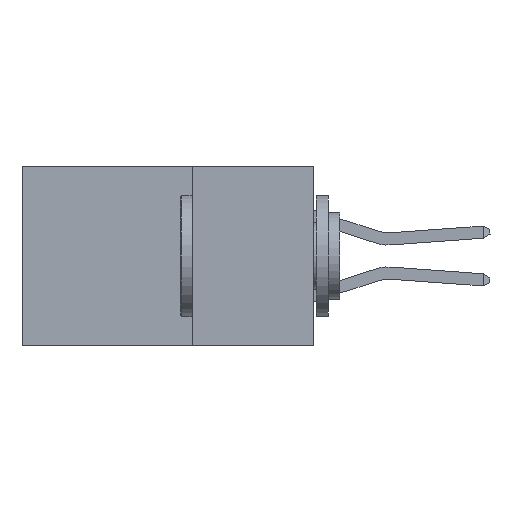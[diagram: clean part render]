
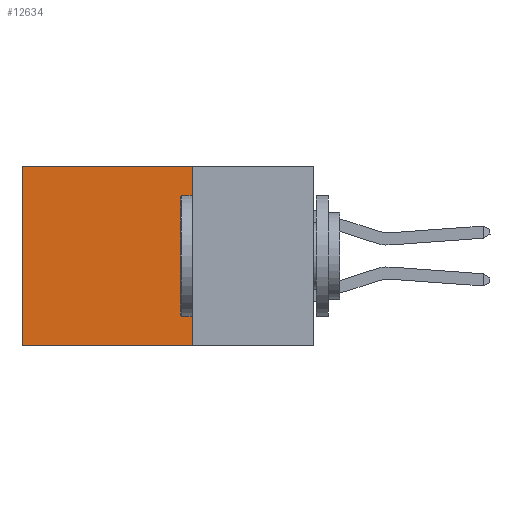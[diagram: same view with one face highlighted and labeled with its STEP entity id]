
A CAD part, left-side view. The second image highlights one B-rep face of the part: STEP entity #12634.
In plain terms, the highlighted planar face has unit normal (-1, 0, 0).
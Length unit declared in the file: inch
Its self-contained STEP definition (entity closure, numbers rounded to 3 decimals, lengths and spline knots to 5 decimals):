
#75 = DIRECTION ( 'NONE',  ( 0., 0., -1. ) ) ;
#630 = LINE ( 'NONE', #6288, #9012 ) ;
#951 = VECTOR ( 'NONE', #9640, 39.37008 ) ;
#1328 = EDGE_CURVE ( 'NONE', #14599, #2252, #17399, .T. ) ;
#1949 = LINE ( 'NONE', #2271, #10211 ) ;
#1964 = FACE_OUTER_BOUND ( 'NONE', #18501, .T. ) ;
#2252 = VERTEX_POINT ( 'NONE', #11704 ) ;
#2271 = CARTESIAN_POINT ( 'NONE',  ( 0.2875, 0.25, -0.37 ) ) ;
#3451 = PLANE ( 'NONE',  #10579 ) ;
#4205 = EDGE_CURVE ( 'NONE', #14599, #5787, #630, .T. ) ;
#4872 = VERTEX_POINT ( 'NONE', #7688 ) ;
#5141 = DIRECTION ( 'NONE',  ( 1., 0., 0. ) ) ;
#5209 = CARTESIAN_POINT ( 'NONE',  ( 0.2875, 0.25, 0. ) ) ;
#5787 = VERTEX_POINT ( 'NONE', #16087 ) ;
#6288 = CARTESIAN_POINT ( 'NONE',  ( 0.2875, 0.25, 0. ) ) ;
#6565 = DIRECTION ( 'NONE',  ( 0., 1., 0. ) ) ;
#7688 = CARTESIAN_POINT ( 'NONE',  ( 0.2875, 0.6, -0.37 ) ) ;
#8024 = CARTESIAN_POINT ( 'NONE',  ( 0.2875, 0.6, 0. ) ) ;
#9012 = VECTOR ( 'NONE', #6565, 39.37008 ) ;
#9640 = DIRECTION ( 'NONE',  ( 0., 0., -1. ) ) ;
#9945 = ORIENTED_EDGE ( 'NONE', *, *, #9954, .T. ) ;
#9954 = EDGE_CURVE ( 'NONE', #5787, #4872, #13933, .T. ) ;
#9970 = CARTESIAN_POINT ( 'NONE',  ( 0.2875, 0.25, 0. ) ) ;
#10211 = VECTOR ( 'NONE', #15088, 39.37008 ) ;
#10579 = AXIS2_PLACEMENT_3D ( 'NONE', #9970, #5141, #16147 ) ;
#11347 = CARTESIAN_POINT ( 'NONE',  ( 0.2875, 0.25, 0. ) ) ;
#11704 = CARTESIAN_POINT ( 'NONE',  ( 0.2875, 0.25, -0.37 ) ) ;
#12634 = ADVANCED_FACE ( 'NONE', ( #1964 ), #3451, .F. ) ;
#12867 = VECTOR ( 'NONE', #75, 39.37008 ) ;
#13328 = ORIENTED_EDGE ( 'NONE', *, *, #4205, .T. ) ;
#13933 = LINE ( 'NONE', #8024, #951 ) ;
#14132 = ORIENTED_EDGE ( 'NONE', *, *, #1328, .F. ) ;
#14599 = VERTEX_POINT ( 'NONE', #11347 ) ;
#15088 = DIRECTION ( 'NONE',  ( 0., 1., 0. ) ) ;
#16087 = CARTESIAN_POINT ( 'NONE',  ( 0.2875, 0.6, 0. ) ) ;
#16147 = DIRECTION ( 'NONE',  ( 0., 0., -1. ) ) ;
#17399 = LINE ( 'NONE', #5209, #12867 ) ;
#18501 = EDGE_LOOP ( 'NONE', ( #9945, #19334, #14132, #13328 ) ) ;
#19334 = ORIENTED_EDGE ( 'NONE', *, *, #20259, .F. ) ;
#20259 = EDGE_CURVE ( 'NONE', #2252, #4872, #1949, .T. ) ;
